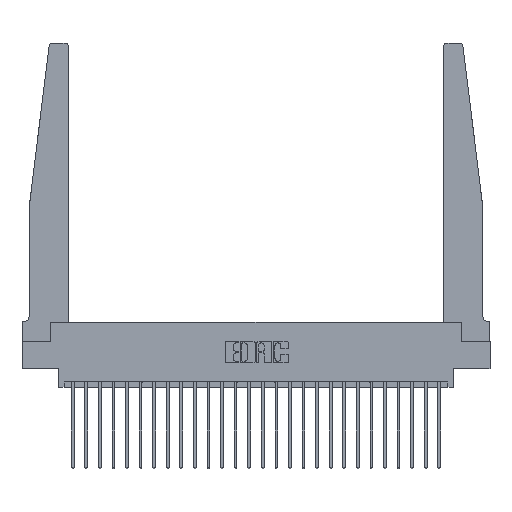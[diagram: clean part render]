
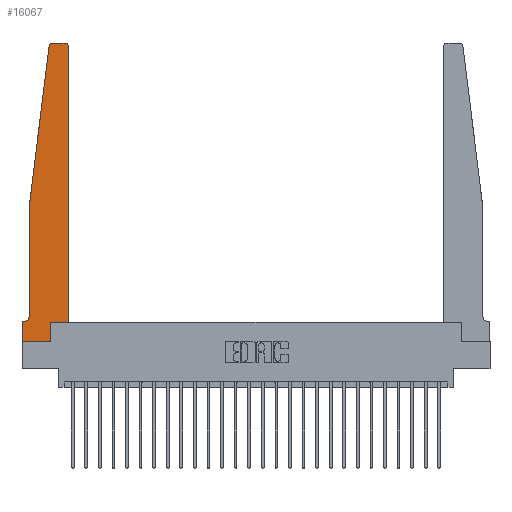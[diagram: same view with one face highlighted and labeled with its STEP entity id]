
A CAD part, top view. The second image highlights one B-rep face of the part: STEP entity #16067.
In plain terms, the highlighted planar face has unit normal (0, 0, 1).
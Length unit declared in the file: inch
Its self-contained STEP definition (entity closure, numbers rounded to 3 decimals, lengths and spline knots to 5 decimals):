
#305 = AXIS2_PLACEMENT_3D ( 'NONE', #5845, #7512, #15167 ) ;
#368 = AXIS2_PLACEMENT_3D ( 'NONE', #13046, #1250, #20896 ) ;
#515 = EDGE_CURVE ( 'NONE', #2543, #21548, #11489, .T. ) ;
#661 = VECTOR ( 'NONE', #11945, 39.37008 ) ;
#1036 = EDGE_CURVE ( 'NONE', #12750, #14254, #14611, .T. ) ;
#1250 = DIRECTION ( 'NONE',  ( 0., 0., -1. ) ) ;
#1259 = PLANE ( 'NONE',  #7210 ) ;
#1492 = LINE ( 'NONE', #9414, #7788 ) ;
#1837 = VECTOR ( 'NONE', #23522, 39.37008 ) ;
#2458 = ORIENTED_EDGE ( 'NONE', *, *, #18390, .T. ) ;
#2543 = VERTEX_POINT ( 'NONE', #4838 ) ;
#2668 = DIRECTION ( 'NONE',  ( -1., 0., 0. ) ) ;
#2880 = VERTEX_POINT ( 'NONE', #7658 ) ;
#3181 = DIRECTION ( 'NONE',  ( 1., 0., 0. ) ) ;
#3329 = ORIENTED_EDGE ( 'NONE', *, *, #22504, .T. ) ;
#3639 = EDGE_CURVE ( 'NONE', #7809, #12750, #16879, .T. ) ;
#3860 = CARTESIAN_POINT ( 'NONE',  ( 0.395, 2.75, 0.37 ) ) ;
#4476 = CARTESIAN_POINT ( 'NONE',  ( 0.425, 2.72, 0.37 ) ) ;
#4594 = VECTOR ( 'NONE', #12771, 39.37008 ) ;
#4838 = CARTESIAN_POINT ( 'NONE',  ( 0.27653, 2.75, 0.37 ) ) ;
#5185 = ORIENTED_EDGE ( 'NONE', *, *, #5746, .T. ) ;
#5552 = EDGE_CURVE ( 'NONE', #21548, #15946, #8438, .T. ) ;
#5746 = EDGE_CURVE ( 'NONE', #10822, #7809, #15676, .T. ) ;
#5845 = CARTESIAN_POINT ( 'NONE',  ( 0.27653, 2.72, 0.37 ) ) ;
#5987 = VECTOR ( 'NONE', #19928, 39.37008 ) ;
#6991 = CARTESIAN_POINT ( 'NONE',  ( 0.065, 1.25, 0.37 ) ) ;
#7209 = CARTESIAN_POINT ( 'NONE',  ( 0., 0.1875, 0.37 ) ) ;
#7210 = AXIS2_PLACEMENT_3D ( 'NONE', #19345, #13328, #11257 ) ;
#7463 = EDGE_LOOP ( 'NONE', ( #3329, #19102, #9424, #19877, #16807, #14284, #2458, #16282, #5185, #25395, #7760, #8270 ) ) ;
#7512 = DIRECTION ( 'NONE',  ( 0., 0., 1. ) ) ;
#7658 = CARTESIAN_POINT ( 'NONE',  ( 0.015, 0.1875, 0.37 ) ) ;
#7760 = ORIENTED_EDGE ( 'NONE', *, *, #1036, .T. ) ;
#7788 = VECTOR ( 'NONE', #3181, 39.37008 ) ;
#7809 = VERTEX_POINT ( 'NONE', #22455 ) ;
#8203 = VERTEX_POINT ( 'NONE', #3860 ) ;
#8270 = ORIENTED_EDGE ( 'NONE', *, *, #10421, .T. ) ;
#8360 = LINE ( 'NONE', #22423, #12018 ) ;
#8438 = LINE ( 'NONE', #16309, #5987 ) ;
#8541 = DIRECTION ( 'NONE',  ( 0., 1., 0. ) ) ;
#8937 = LINE ( 'NONE', #6991, #24989 ) ;
#9367 = CARTESIAN_POINT ( 'NONE',  ( 0.2605, 0.18, 0.37 ) ) ;
#9414 = CARTESIAN_POINT ( 'NONE',  ( 0., 0., 0.37 ) ) ;
#9424 = ORIENTED_EDGE ( 'NONE', *, *, #5552, .T. ) ;
#9835 = AXIS2_PLACEMENT_3D ( 'NONE', #10029, #12683, #10754 ) ;
#10029 = CARTESIAN_POINT ( 'NONE',  ( 0.395, 2.72, 0.37 ) ) ;
#10421 = EDGE_CURVE ( 'NONE', #14254, #8203, #20937, .T. ) ;
#10489 = CARTESIAN_POINT ( 'NONE',  ( 0.065, 1.25, 0.37 ) ) ;
#10754 = DIRECTION ( 'NONE',  ( 1., 0., 0. ) ) ;
#10822 = VERTEX_POINT ( 'NONE', #15017 ) ;
#10965 = CARTESIAN_POINT ( 'NONE',  ( 0.425, 0.18, 0.37 ) ) ;
#11126 = VECTOR ( 'NONE', #8541, 39.37008 ) ;
#11176 = VERTEX_POINT ( 'NONE', #16378 ) ;
#11257 = DIRECTION ( 'NONE',  ( 1., 0., 0. ) ) ;
#11489 = CIRCLE ( 'NONE', #305, 0.03 ) ;
#11499 = VECTOR ( 'NONE', #14602, 39.37008 ) ;
#11565 = CIRCLE ( 'NONE', #368, 0.05 ) ;
#11945 = DIRECTION ( 'NONE',  ( 0., -1., 0. ) ) ;
#12018 = VECTOR ( 'NONE', #2668, 39.37008 ) ;
#12071 = EDGE_CURVE ( 'NONE', #15946, #11176, #8937, .T. ) ;
#12683 = DIRECTION ( 'NONE',  ( 0., 0., 1. ) ) ;
#12750 = VERTEX_POINT ( 'NONE', #20096 ) ;
#12771 = DIRECTION ( 'NONE',  ( 1., 0., 0. ) ) ;
#13046 = CARTESIAN_POINT ( 'NONE',  ( 0.015, 0.2375, 0.37 ) ) ;
#13058 = LINE ( 'NONE', #16909, #11499 ) ;
#13328 = DIRECTION ( 'NONE',  ( 0., 0., 1. ) ) ;
#14254 = VERTEX_POINT ( 'NONE', #4476 ) ;
#14284 = ORIENTED_EDGE ( 'NONE', *, *, #15027, .T. ) ;
#14602 = DIRECTION ( 'NONE',  ( -1., 0., 0. ) ) ;
#14611 = LINE ( 'NONE', #20797, #11126 ) ;
#14820 = CARTESIAN_POINT ( 'NONE',  ( 0., 0., 0.37 ) ) ;
#14900 = DIRECTION ( 'NONE',  ( 0., -1., 0. ) ) ;
#15017 = CARTESIAN_POINT ( 'NONE',  ( 0.2605, 0., 0.37 ) ) ;
#15027 = EDGE_CURVE ( 'NONE', #2880, #24357, #8360, .T. ) ;
#15127 = EDGE_CURVE ( 'NONE', #18052, #10822, #1492, .T. ) ;
#15167 = DIRECTION ( 'NONE',  ( 1., 0., 0. ) ) ;
#15676 = LINE ( 'NONE', #9367, #1837 ) ;
#15946 = VERTEX_POINT ( 'NONE', #10489 ) ;
#16067 = ADVANCED_FACE ( 'NONE', ( #21285 ), #1259, .T. ) ;
#16105 = CARTESIAN_POINT ( 'NONE',  ( 0.24675, 2.72367, 0.37 ) ) ;
#16282 = ORIENTED_EDGE ( 'NONE', *, *, #15127, .T. ) ;
#16309 = CARTESIAN_POINT ( 'NONE',  ( 0.065, 1.25, 0.37 ) ) ;
#16378 = CARTESIAN_POINT ( 'NONE',  ( 0.065, 0.2375, 0.37 ) ) ;
#16807 = ORIENTED_EDGE ( 'NONE', *, *, #24365, .T. ) ;
#16879 = LINE ( 'NONE', #10965, #4594 ) ;
#16909 = CARTESIAN_POINT ( 'NONE',  ( 0.25, 2.75, 0.37 ) ) ;
#18052 = VERTEX_POINT ( 'NONE', #14820 ) ;
#18390 = EDGE_CURVE ( 'NONE', #24357, #18052, #23933, .T. ) ;
#19102 = ORIENTED_EDGE ( 'NONE', *, *, #515, .T. ) ;
#19345 = CARTESIAN_POINT ( 'NONE',  ( 0., 0.1875, 0.37 ) ) ;
#19669 = CARTESIAN_POINT ( 'NONE',  ( 0., 0., 0.37 ) ) ;
#19877 = ORIENTED_EDGE ( 'NONE', *, *, #12071, .T. ) ;
#19928 = DIRECTION ( 'NONE',  ( -0.122, -0.992, 0. ) ) ;
#20096 = CARTESIAN_POINT ( 'NONE',  ( 0.425, 0.18, 0.37 ) ) ;
#20797 = CARTESIAN_POINT ( 'NONE',  ( 0.425, 0.18, 0.37 ) ) ;
#20896 = DIRECTION ( 'NONE',  ( -1., 0., 0. ) ) ;
#20937 = CIRCLE ( 'NONE', #9835, 0.03 ) ;
#21285 = FACE_OUTER_BOUND ( 'NONE', #7463, .T. ) ;
#21548 = VERTEX_POINT ( 'NONE', #16105 ) ;
#22423 = CARTESIAN_POINT ( 'NONE',  ( 0.065, 0.1875, 0.37 ) ) ;
#22455 = CARTESIAN_POINT ( 'NONE',  ( 0.2605, 0.18, 0.37 ) ) ;
#22504 = EDGE_CURVE ( 'NONE', #8203, #2543, #13058, .T. ) ;
#23522 = DIRECTION ( 'NONE',  ( 0., 1., 0. ) ) ;
#23933 = LINE ( 'NONE', #19669, #661 ) ;
#24357 = VERTEX_POINT ( 'NONE', #7209 ) ;
#24365 = EDGE_CURVE ( 'NONE', #11176, #2880, #11565, .T. ) ;
#24989 = VECTOR ( 'NONE', #14900, 39.37008 ) ;
#25395 = ORIENTED_EDGE ( 'NONE', *, *, #3639, .T. ) ;
